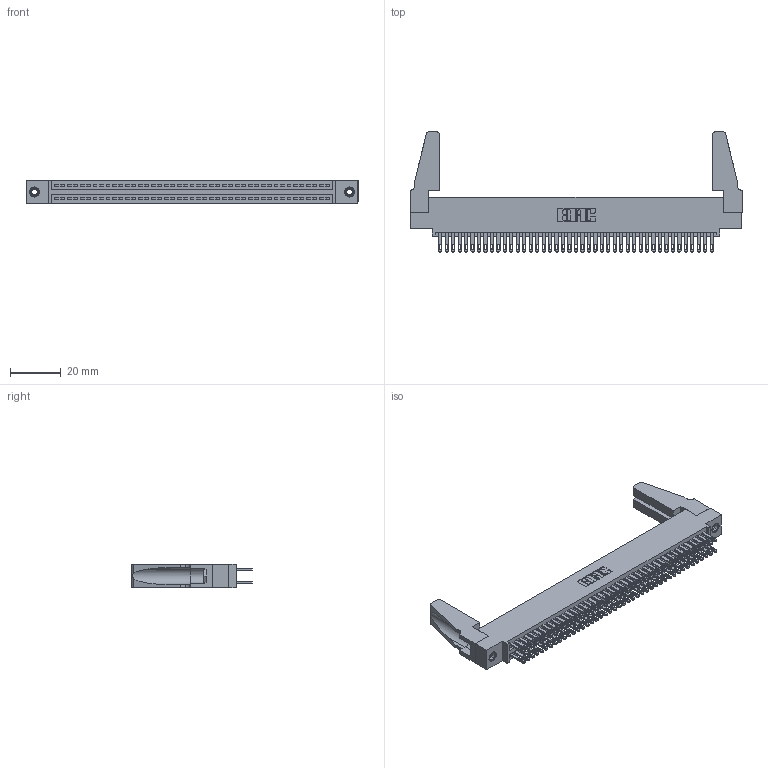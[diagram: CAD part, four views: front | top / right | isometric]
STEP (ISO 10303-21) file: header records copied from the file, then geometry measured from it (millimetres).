
FILE_DESCRIPTION (( 'STEP AP203' ), '1' );
FILE_NAME ('345-086-500-588.STEP', '2019-11-01T06:21:13', ( '' ), ( '' ), 'SwSTEP 2.0', 'SolidWorks 2016', '' );
FILE_SCHEMA (( 'CONFIG_CONTROL_DESIGN' ));
Length unit declared in the file: inch
Products named in the file (5): 345-086-500-588; 345-292-001_345-293-100; 345-250-001_345-250-001-102; 345 Part_0.110 Offset - 0.156 Dia-TH; 345-220-078_345-220-088
Assembly tree (91 placements, depth 2):
  345-086-500-588
    345 Part_0.110 Offset - 0.156 Dia-TH
    345-292-001_345-293-100  x86
    345-250-001_345-250-001-102  x2
    345-220-078_345-220-088  x2
Bounding box: 130.45 x 47.17 x 9.4 mm (x, y, z)
Volume: 16123.6 mm3; surface area: 23137.3 mm2
Topology: 91 solids, 91 shells, 4210 faces, 12793 edges, 8518 vertices
Faces by surface type: plane 2478, cylinder 1716, cone 12, torus 4
Entity records: 35814 total; most frequent: CARTESIAN_POINT 5998, ORIENTED_EDGE 5892, DIRECTION 5294, EDGE_CURVE 2946, VECTOR 2596, LINE 2596, VERTEX_POINT 1958, AXIS2_PLACEMENT_3D 1349
